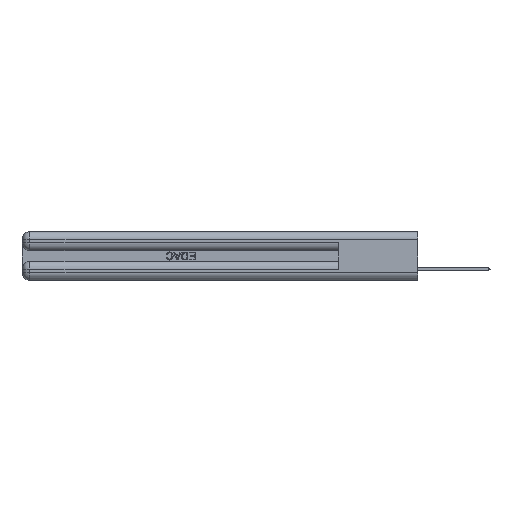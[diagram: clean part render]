
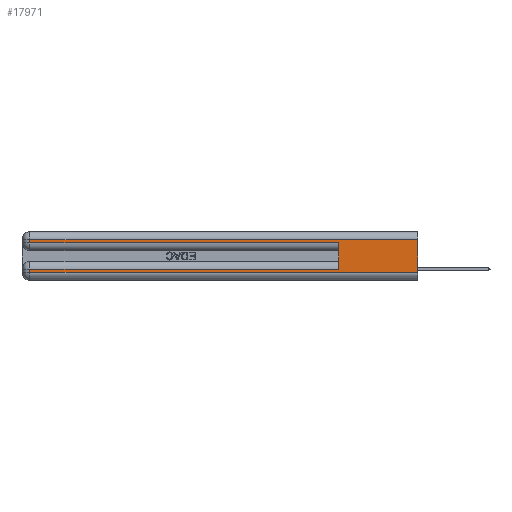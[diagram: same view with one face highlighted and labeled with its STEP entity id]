
A CAD part, left-side view. The second image highlights one B-rep face of the part: STEP entity #17971.
In plain terms, the highlighted planar face has unit normal (-1, 0, 0).
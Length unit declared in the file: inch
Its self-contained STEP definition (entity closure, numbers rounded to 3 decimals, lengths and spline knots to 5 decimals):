
#640 = CARTESIAN_POINT ( 'NONE',  ( 0., 2.94, 0.37 ) ) ;
#712 = LINE ( 'NONE', #29758, #51071 ) ;
#875 = LINE ( 'NONE', #52867, #5303 ) ;
#1150 = EDGE_CURVE ( 'NONE', #1892, #38604, #20261, .T. ) ;
#1632 = ORIENTED_EDGE ( 'NONE', *, *, #4532, .T. ) ;
#1892 = VERTEX_POINT ( 'NONE', #43177 ) ;
#2063 = CARTESIAN_POINT ( 'NONE',  ( 0., 2.94, 0.06 ) ) ;
#2262 = CARTESIAN_POINT ( 'NONE',  ( 0., 0., 0.31 ) ) ;
#4499 = ORIENTED_EDGE ( 'NONE', *, *, #42431, .F. ) ;
#4532 = EDGE_CURVE ( 'NONE', #42237, #16351, #9817, .T. ) ;
#5303 = VECTOR ( 'NONE', #48888, 39.37008 ) ;
#9038 = LINE ( 'NONE', #14978, #15550 ) ;
#9624 = PLANE ( 'NONE',  #46238 ) ;
#9817 = LINE ( 'NONE', #18114, #15464 ) ;
#9969 = CARTESIAN_POINT ( 'NONE',  ( 0., 0., 0.37 ) ) ;
#11344 = DIRECTION ( 'NONE',  ( 0., 0., 1. ) ) ;
#14081 = CARTESIAN_POINT ( 'NONE',  ( 0., 2.94, 0.285 ) ) ;
#14159 = DIRECTION ( 'NONE',  ( 1., 0., 0. ) ) ;
#14370 = DIRECTION ( 'NONE',  ( 0., 0., -1. ) ) ;
#14978 = CARTESIAN_POINT ( 'NONE',  ( 0., 0., 0.37 ) ) ;
#15464 = VECTOR ( 'NONE', #37890, 39.37008 ) ;
#15550 = VECTOR ( 'NONE', #31289, 39.37008 ) ;
#16351 = VERTEX_POINT ( 'NONE', #46858 ) ;
#16603 = VECTOR ( 'NONE', #26886, 39.37008 ) ;
#17838 = FACE_OUTER_BOUND ( 'NONE', #31749, .T. ) ;
#17957 = DIRECTION ( 'NONE',  ( 0., 0., -1. ) ) ;
#17971 = ADVANCED_FACE ( 'NONE', ( #17838 ), #9624, .F. ) ;
#18114 = CARTESIAN_POINT ( 'NONE',  ( 0., 0., 0.285 ) ) ;
#18938 = CARTESIAN_POINT ( 'NONE',  ( 0., 0.6, 0.085 ) ) ;
#20261 = LINE ( 'NONE', #640, #22856 ) ;
#22319 = VERTEX_POINT ( 'NONE', #18938 ) ;
#22856 = VECTOR ( 'NONE', #50651, 39.37008 ) ;
#26566 = ORIENTED_EDGE ( 'NONE', *, *, #29756, .T. ) ;
#26886 = DIRECTION ( 'NONE',  ( 0., -1., 0. ) ) ;
#27856 = CARTESIAN_POINT ( 'NONE',  ( 0., 0.6, 0.145 ) ) ;
#29403 = CARTESIAN_POINT ( 'NONE',  ( 0., 2.94, 0.31 ) ) ;
#29756 = EDGE_CURVE ( 'NONE', #33284, #43364, #875, .T. ) ;
#29758 = CARTESIAN_POINT ( 'NONE',  ( 0., 0., 0.085 ) ) ;
#31289 = DIRECTION ( 'NONE',  ( 0., 0., -1. ) ) ;
#31749 = EDGE_LOOP ( 'NONE', ( #36190, #26566, #35731, #1632, #4499, #36054, #46416, #36660 ) ) ;
#33214 = EDGE_CURVE ( 'NONE', #38604, #38408, #46378, .T. ) ;
#33284 = VERTEX_POINT ( 'NONE', #2262 ) ;
#35047 = CARTESIAN_POINT ( 'NONE',  ( 0., 0., 0.06 ) ) ;
#35731 = ORIENTED_EDGE ( 'NONE', *, *, #52557, .T. ) ;
#36054 = ORIENTED_EDGE ( 'NONE', *, *, #37295, .T. ) ;
#36190 = ORIENTED_EDGE ( 'NONE', *, *, #53175, .F. ) ;
#36660 = ORIENTED_EDGE ( 'NONE', *, *, #33214, .T. ) ;
#37295 = EDGE_CURVE ( 'NONE', #22319, #1892, #712, .T. ) ;
#37890 = DIRECTION ( 'NONE',  ( 0., -1., 0. ) ) ;
#38289 = VECTOR ( 'NONE', #14370, 39.37008 ) ;
#38408 = VERTEX_POINT ( 'NONE', #46043 ) ;
#38604 = VERTEX_POINT ( 'NONE', #2063 ) ;
#39142 = CARTESIAN_POINT ( 'NONE',  ( 0., 2.94, 0.37 ) ) ;
#41721 = VECTOR ( 'NONE', #11344, 39.37008 ) ;
#42237 = VERTEX_POINT ( 'NONE', #14081 ) ;
#42431 = EDGE_CURVE ( 'NONE', #22319, #16351, #44917, .T. ) ;
#43177 = CARTESIAN_POINT ( 'NONE',  ( 0., 2.94, 0.085 ) ) ;
#43364 = VERTEX_POINT ( 'NONE', #29403 ) ;
#44917 = LINE ( 'NONE', #27856, #41721 ) ;
#45817 = DIRECTION ( 'NONE',  ( 0., 1., 0. ) ) ;
#46043 = CARTESIAN_POINT ( 'NONE',  ( 0., 0., 0.06 ) ) ;
#46238 = AXIS2_PLACEMENT_3D ( 'NONE', #9969, #14159, #17957 ) ;
#46378 = LINE ( 'NONE', #35047, #16603 ) ;
#46416 = ORIENTED_EDGE ( 'NONE', *, *, #1150, .T. ) ;
#46858 = CARTESIAN_POINT ( 'NONE',  ( 0., 0.6, 0.285 ) ) ;
#47946 = LINE ( 'NONE', #39142, #38289 ) ;
#48888 = DIRECTION ( 'NONE',  ( 0., 1., 0. ) ) ;
#50651 = DIRECTION ( 'NONE',  ( 0., 0., -1. ) ) ;
#51071 = VECTOR ( 'NONE', #45817, 39.37008 ) ;
#52557 = EDGE_CURVE ( 'NONE', #43364, #42237, #47946, .T. ) ;
#52867 = CARTESIAN_POINT ( 'NONE',  ( 0., 0., 0.31 ) ) ;
#53175 = EDGE_CURVE ( 'NONE', #33284, #38408, #9038, .T. ) ;
